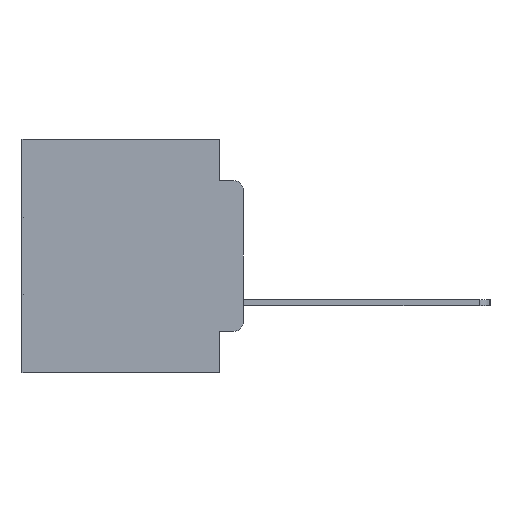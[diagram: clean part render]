
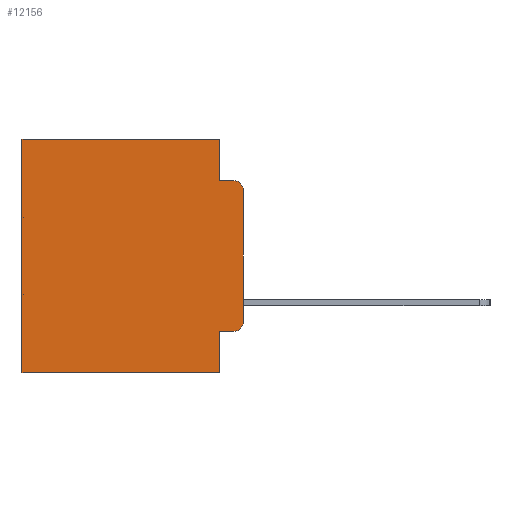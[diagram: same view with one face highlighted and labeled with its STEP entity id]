
A CAD part, left-side view. The second image highlights one B-rep face of the part: STEP entity #12156.
In plain terms, the highlighted planar face has unit normal (-1, 0, 0).
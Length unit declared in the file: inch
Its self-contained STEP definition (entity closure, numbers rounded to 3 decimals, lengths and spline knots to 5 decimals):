
#1470 = VECTOR ( 'NONE', #13640, 39.37008 ) ;
#2001 = LINE ( 'NONE', #25601, #26669 ) ;
#3190 = CARTESIAN_POINT ( 'NONE',  ( 0.298, 0.051, 0. ) ) ;
#3517 = CARTESIAN_POINT ( 'NONE',  ( 0.298, 0., -0.3915 ) ) ;
#4207 = VERTEX_POINT ( 'NONE', #24911 ) ;
#4939 = CARTESIAN_POINT ( 'NONE',  ( 0.298, 0.473, 0. ) ) ;
#5136 = VERTEX_POINT ( 'NONE', #27207 ) ;
#5301 = PLANE ( 'NONE',  #29924 ) ;
#5535 = DIRECTION ( 'NONE',  ( 0., 0., -1. ) ) ;
#5590 = CIRCLE ( 'NONE', #23319, 0.02 ) ;
#7143 = EDGE_CURVE ( 'NONE', #22022, #4207, #29351, .T. ) ;
#7314 = LINE ( 'NONE', #20623, #19726 ) ;
#7361 = LINE ( 'NONE', #15209, #24647 ) ;
#7953 = DIRECTION ( 'NONE',  ( 0., -1., 0. ) ) ;
#8024 = VERTEX_POINT ( 'NONE', #4939 ) ;
#8109 = CARTESIAN_POINT ( 'NONE',  ( 0.298, 0.02, -0.3915 ) ) ;
#8409 = CARTESIAN_POINT ( 'NONE',  ( 0.298, 0., -0.1085 ) ) ;
#8429 = ORIENTED_EDGE ( 'NONE', *, *, #20270, .T. ) ;
#8558 = LINE ( 'NONE', #14032, #20948 ) ;
#9954 = ORIENTED_EDGE ( 'NONE', *, *, #18215, .T. ) ;
#10111 = DIRECTION ( 'NONE',  ( -1., 0., 0. ) ) ;
#10362 = DIRECTION ( 'NONE',  ( 1., 0., 0. ) ) ;
#10480 = CARTESIAN_POINT ( 'NONE',  ( 0.298, 0.051, 0. ) ) ;
#10585 = DIRECTION ( 'NONE',  ( 0., 0., -1. ) ) ;
#11133 = CARTESIAN_POINT ( 'NONE',  ( 0.298, 0.051, 0. ) ) ;
#11147 = ORIENTED_EDGE ( 'NONE', *, *, #29122, .F. ) ;
#12156 = ADVANCED_FACE ( 'NONE', ( #17827 ), #5301, .F. ) ;
#12218 = CARTESIAN_POINT ( 'NONE',  ( 0.298, 0.051, -0.0885 ) ) ;
#12652 = VERTEX_POINT ( 'NONE', #24500 ) ;
#12681 = ORIENTED_EDGE ( 'NONE', *, *, #23855, .T. ) ;
#12912 = VERTEX_POINT ( 'NONE', #3190 ) ;
#13640 = DIRECTION ( 'NONE',  ( 0., 0., -1. ) ) ;
#14032 = CARTESIAN_POINT ( 'NONE',  ( 0.298, 0., 0. ) ) ;
#15067 = ORIENTED_EDGE ( 'NONE', *, *, #7143, .F. ) ;
#15209 = CARTESIAN_POINT ( 'NONE',  ( 0.298, 0.473, 0. ) ) ;
#15839 = ORIENTED_EDGE ( 'NONE', *, *, #22466, .F. ) ;
#16616 = ORIENTED_EDGE ( 'NONE', *, *, #30629, .T. ) ;
#17675 = DIRECTION ( 'NONE',  ( 0., 0., -1. ) ) ;
#17748 = ORIENTED_EDGE ( 'NONE', *, *, #19287, .F. ) ;
#17810 = EDGE_LOOP ( 'NONE', ( #22660, #29731, #11147, #17748, #12681, #8429, #15067, #15839, #9954, #16616 ) ) ;
#17827 = FACE_OUTER_BOUND ( 'NONE', #17810, .T. ) ;
#18135 = CARTESIAN_POINT ( 'NONE',  ( 0.298, 0.051, -0.5 ) ) ;
#18215 = EDGE_CURVE ( 'NONE', #23581, #12652, #7314, .T. ) ;
#19287 = EDGE_CURVE ( 'NONE', #12912, #20769, #27681, .T. ) ;
#19726 = VECTOR ( 'NONE', #23037, 39.37008 ) ;
#19971 = EDGE_CURVE ( 'NONE', #26093, #27501, #8558, .T. ) ;
#20270 = EDGE_CURVE ( 'NONE', #8024, #4207, #7361, .T. ) ;
#20304 = CARTESIAN_POINT ( 'NONE',  ( 0.298, 0.051, -0.0885 ) ) ;
#20446 = LINE ( 'NONE', #20304, #26050 ) ;
#20517 = AXIS2_PLACEMENT_3D ( 'NONE', #24820, #10111, #27187 ) ;
#20623 = CARTESIAN_POINT ( 'NONE',  ( 0.298, 0.051, -0.4115 ) ) ;
#20769 = VERTEX_POINT ( 'NONE', #12218 ) ;
#20804 = DIRECTION ( 'NONE',  ( 0., 1., 0. ) ) ;
#20862 = CARTESIAN_POINT ( 'NONE',  ( 0.298, 0., -0.5 ) ) ;
#20948 = VECTOR ( 'NONE', #21226, 39.37008 ) ;
#21226 = DIRECTION ( 'NONE',  ( 0., 0., -1. ) ) ;
#21930 = VECTOR ( 'NONE', #5535, 39.37008 ) ;
#22022 = VERTEX_POINT ( 'NONE', #18135 ) ;
#22466 = EDGE_CURVE ( 'NONE', #23581, #22022, #28262, .T. ) ;
#22660 = ORIENTED_EDGE ( 'NONE', *, *, #19971, .F. ) ;
#23037 = DIRECTION ( 'NONE',  ( 0., -1., 0. ) ) ;
#23319 = AXIS2_PLACEMENT_3D ( 'NONE', #8109, #25260, #10585 ) ;
#23581 = VERTEX_POINT ( 'NONE', #24680 ) ;
#23855 = EDGE_CURVE ( 'NONE', #12912, #8024, #2001, .T. ) ;
#24500 = CARTESIAN_POINT ( 'NONE',  ( 0.298, 0.02, -0.4115 ) ) ;
#24647 = VECTOR ( 'NONE', #17675, 39.37008 ) ;
#24680 = CARTESIAN_POINT ( 'NONE',  ( 0.298, 0.051, -0.4115 ) ) ;
#24820 = CARTESIAN_POINT ( 'NONE',  ( 0.298, 0.02, -0.1085 ) ) ;
#24911 = CARTESIAN_POINT ( 'NONE',  ( 0.298, 0.473, -0.5 ) ) ;
#25260 = DIRECTION ( 'NONE',  ( -1., 0., 0. ) ) ;
#25601 = CARTESIAN_POINT ( 'NONE',  ( 0.298, 0., 0. ) ) ;
#25627 = CIRCLE ( 'NONE', #20517, 0.02 ) ;
#25651 = DIRECTION ( 'NONE',  ( 0., 1., 0. ) ) ;
#26050 = VECTOR ( 'NONE', #7953, 39.37008 ) ;
#26093 = VERTEX_POINT ( 'NONE', #8409 ) ;
#26669 = VECTOR ( 'NONE', #20804, 39.37008 ) ;
#27187 = DIRECTION ( 'NONE',  ( 0., 0., -1. ) ) ;
#27207 = CARTESIAN_POINT ( 'NONE',  ( 0.298, 0.02, -0.0885 ) ) ;
#27431 = DIRECTION ( 'NONE',  ( 0., 0., -1. ) ) ;
#27501 = VERTEX_POINT ( 'NONE', #3517 ) ;
#27681 = LINE ( 'NONE', #11133, #1470 ) ;
#28262 = LINE ( 'NONE', #10480, #21930 ) ;
#28606 = VECTOR ( 'NONE', #25651, 39.37008 ) ;
#29122 = EDGE_CURVE ( 'NONE', #20769, #5136, #20446, .T. ) ;
#29351 = LINE ( 'NONE', #20862, #28606 ) ;
#29718 = CARTESIAN_POINT ( 'NONE',  ( 0.298, 0., 0. ) ) ;
#29731 = ORIENTED_EDGE ( 'NONE', *, *, #31138, .T. ) ;
#29924 = AXIS2_PLACEMENT_3D ( 'NONE', #29718, #10362, #27431 ) ;
#30629 = EDGE_CURVE ( 'NONE', #12652, #27501, #5590, .T. ) ;
#31138 = EDGE_CURVE ( 'NONE', #26093, #5136, #25627, .T. ) ;
